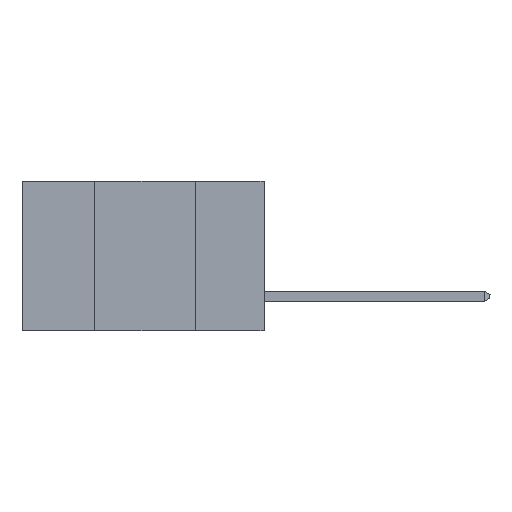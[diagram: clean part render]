
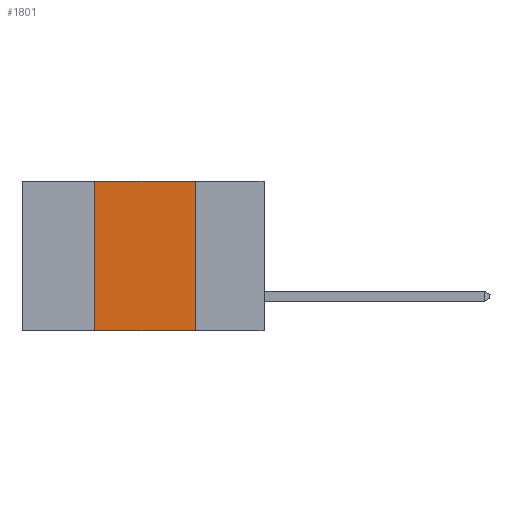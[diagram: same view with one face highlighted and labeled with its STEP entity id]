
A CAD part, left-side view. The second image highlights one B-rep face of the part: STEP entity #1801.
In plain terms, the highlighted planar face has unit normal (-1, 0, 0).
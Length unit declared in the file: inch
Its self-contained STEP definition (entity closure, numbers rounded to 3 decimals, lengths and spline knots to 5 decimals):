
#433 = DIRECTION ( 'NONE',  ( 0., -1., 0. ) ) ;
#899 = LINE ( 'NONE', #14150, #14535 ) ;
#978 = CARTESIAN_POINT ( 'NONE',  ( 0., 0.6, 0. ) ) ;
#1124 = VERTEX_POINT ( 'NONE', #14178 ) ;
#1407 = VECTOR ( 'NONE', #16809, 39.37008 ) ;
#1463 = ORIENTED_EDGE ( 'NONE', *, *, #11750, .F. ) ;
#1801 = ADVANCED_FACE ( 'NONE', ( #11632 ), #13989, .F. ) ;
#1916 = VERTEX_POINT ( 'NONE', #8762 ) ;
#2206 = EDGE_LOOP ( 'NONE', ( #1463, #6253, #3536, #7613 ) ) ;
#3536 = ORIENTED_EDGE ( 'NONE', *, *, #16410, .F. ) ;
#4456 = CARTESIAN_POINT ( 'NONE',  ( 0., 0.17, -0.37 ) ) ;
#5103 = LINE ( 'NONE', #978, #12260 ) ;
#5478 = CARTESIAN_POINT ( 'NONE',  ( 0., 0.6, 0. ) ) ;
#6253 = ORIENTED_EDGE ( 'NONE', *, *, #13159, .F. ) ;
#6844 = DIRECTION ( 'NONE',  ( 0., 0., -1. ) ) ;
#6856 = EDGE_CURVE ( 'NONE', #1124, #14515, #17376, .T. ) ;
#7028 = VERTEX_POINT ( 'NONE', #12999 ) ;
#7343 = VECTOR ( 'NONE', #433, 39.37008 ) ;
#7613 = ORIENTED_EDGE ( 'NONE', *, *, #6856, .T. ) ;
#8489 = DIRECTION ( 'NONE',  ( 0., 0., -1. ) ) ;
#8762 = CARTESIAN_POINT ( 'NONE',  ( 0., 0.42, 0. ) ) ;
#9848 = AXIS2_PLACEMENT_3D ( 'NONE', #5478, #15335, #6844 ) ;
#11289 = DIRECTION ( 'NONE',  ( 0., -1., 0. ) ) ;
#11632 = FACE_OUTER_BOUND ( 'NONE', #2206, .T. ) ;
#11750 = EDGE_CURVE ( 'NONE', #7028, #14515, #899, .T. ) ;
#12260 = VECTOR ( 'NONE', #11289, 39.37008 ) ;
#12999 = CARTESIAN_POINT ( 'NONE',  ( 0., 0.17, 0. ) ) ;
#13159 = EDGE_CURVE ( 'NONE', #1916, #7028, #5103, .T. ) ;
#13966 = LINE ( 'NONE', #15575, #1407 ) ;
#13989 = PLANE ( 'NONE',  #9848 ) ;
#14150 = CARTESIAN_POINT ( 'NONE',  ( 0., 0.17, 0. ) ) ;
#14178 = CARTESIAN_POINT ( 'NONE',  ( 0., 0.42, -0.37 ) ) ;
#14515 = VERTEX_POINT ( 'NONE', #4456 ) ;
#14535 = VECTOR ( 'NONE', #8489, 39.37008 ) ;
#15335 = DIRECTION ( 'NONE',  ( 1., 0., 0. ) ) ;
#15575 = CARTESIAN_POINT ( 'NONE',  ( 0., 0.42, 0. ) ) ;
#16410 = EDGE_CURVE ( 'NONE', #1124, #1916, #13966, .T. ) ;
#16809 = DIRECTION ( 'NONE',  ( 0., 0., 1. ) ) ;
#17376 = LINE ( 'NONE', #17765, #7343 ) ;
#17765 = CARTESIAN_POINT ( 'NONE',  ( 0., 0.6, -0.37 ) ) ;
